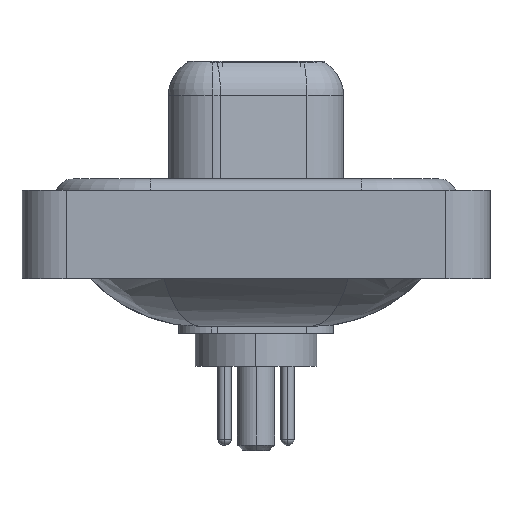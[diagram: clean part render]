
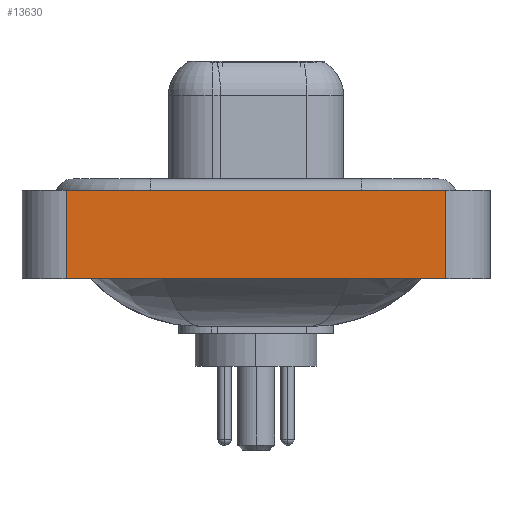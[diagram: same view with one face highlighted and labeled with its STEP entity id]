
A CAD part, left-side view. The second image highlights one B-rep face of the part: STEP entity #13630.
In plain terms, the highlighted planar face has unit normal (-1, 0, 0).
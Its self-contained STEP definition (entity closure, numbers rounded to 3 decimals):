
#471 = EDGE_CURVE ( 'NONE', #1721, #21712, #11844, .T. ) ;
#513 = DIRECTION ( 'NONE',  ( 0., -1., 0. ) ) ;
#604 = ORIENTED_EDGE ( 'NONE', *, *, #16964, .F. ) ;
#738 = CARTESIAN_POINT ( 'NONE',  ( -7.35, -8.55, -3.6 ) ) ;
#921 = ORIENTED_EDGE ( 'NONE', *, *, #471, .T. ) ;
#1179 = VERTEX_POINT ( 'NONE', #10457 ) ;
#1721 = VERTEX_POINT ( 'NONE', #17345 ) ;
#2045 = DIRECTION ( 'NONE',  ( -1., 0., 0. ) ) ;
#2067 = VERTEX_POINT ( 'NONE', #9098 ) ;
#2181 = VECTOR ( 'NONE', #17712, 1000. ) ;
#2356 = CARTESIAN_POINT ( 'NONE',  ( -7.35, -8.55, 0.4 ) ) ;
#2819 = EDGE_CURVE ( 'NONE', #1179, #1721, #4702, .T. ) ;
#3973 = VECTOR ( 'NONE', #19119, 1000. ) ;
#4702 = LINE ( 'NONE', #738, #18433 ) ;
#6504 = CARTESIAN_POINT ( 'NONE',  ( -7.35, -8.55, -3.6 ) ) ;
#7651 = LINE ( 'NONE', #8028, #3973 ) ;
#7883 = EDGE_LOOP ( 'NONE', ( #921, #14939, #604, #13856 ) ) ;
#8028 = CARTESIAN_POINT ( 'NONE',  ( -7.35, 8.55, -3.6 ) ) ;
#8548 = DIRECTION ( 'NONE',  ( 0., -1., 0. ) ) ;
#8947 = CARTESIAN_POINT ( 'NONE',  ( -7.35, -8.55, 0.4 ) ) ;
#9098 = CARTESIAN_POINT ( 'NONE',  ( -7.35, 8.55, 0.4 ) ) ;
#9153 = AXIS2_PLACEMENT_3D ( 'NONE', #21096, #2045, #18595 ) ;
#10457 = CARTESIAN_POINT ( 'NONE',  ( -7.35, 8.55, -3.6 ) ) ;
#11844 = LINE ( 'NONE', #6504, #2181 ) ;
#12242 = EDGE_CURVE ( 'NONE', #2067, #21712, #15559, .T. ) ;
#13630 = ADVANCED_FACE ( 'NONE', ( #18961 ), #15241, .T. ) ;
#13856 = ORIENTED_EDGE ( 'NONE', *, *, #2819, .T. ) ;
#14939 = ORIENTED_EDGE ( 'NONE', *, *, #12242, .F. ) ;
#15241 = PLANE ( 'NONE',  #9153 ) ;
#15559 = LINE ( 'NONE', #2356, #17467 ) ;
#16964 = EDGE_CURVE ( 'NONE', #1179, #2067, #7651, .T. ) ;
#17345 = CARTESIAN_POINT ( 'NONE',  ( -7.35, -8.55, -3.6 ) ) ;
#17467 = VECTOR ( 'NONE', #513, 1000. ) ;
#17712 = DIRECTION ( 'NONE',  ( 0., 0., 1. ) ) ;
#18433 = VECTOR ( 'NONE', #8548, 1000. ) ;
#18595 = DIRECTION ( 'NONE',  ( 0., 0., 1. ) ) ;
#18961 = FACE_OUTER_BOUND ( 'NONE', #7883, .T. ) ;
#19119 = DIRECTION ( 'NONE',  ( 0., 0., 1. ) ) ;
#21096 = CARTESIAN_POINT ( 'NONE',  ( -7.35, -8.55, -3.6 ) ) ;
#21712 = VERTEX_POINT ( 'NONE', #8947 ) ;
